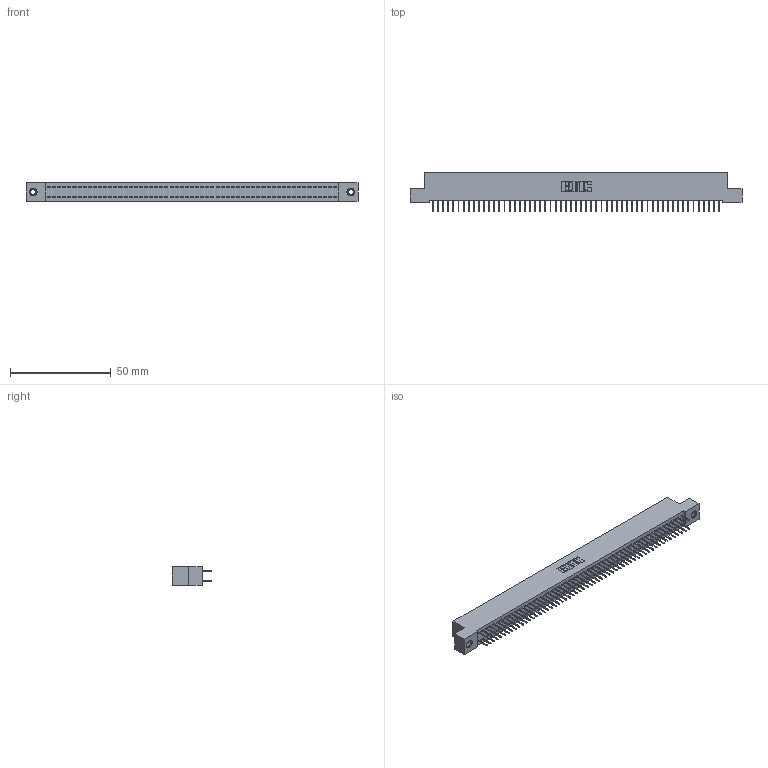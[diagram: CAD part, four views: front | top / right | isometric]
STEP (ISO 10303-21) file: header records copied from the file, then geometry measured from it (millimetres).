
FILE_DESCRIPTION (( 'STEP AP203' ), '1' );
FILE_NAME ('392-114-524-207.STEP', '2019-10-10T00:59:07', ( '' ), ( '' ), 'SwSTEP 2.0', 'SolidWorks 2016', '' );
FILE_SCHEMA (( 'CONFIG_CONTROL_DESIGN' ));
Length unit declared in the file: inch
Products named in the file (4): 345-250-001_345-250-005-103; 392-114-524-207; 342 Part_TI; 345-292-001_345-293-124
Assembly tree (117 placements, depth 2):
  392-114-524-207
    342 Part_TI
    345-292-001_345-293-124  x114
    345-250-001_345-250-005-103  x2
Bounding box: 165.1 x 19.69 x 9.4 mm (x, y, z)
Volume: 14720 mm3; surface area: 23907.1 mm2
Topology: 117 solids, 117 shells, 6554 faces, 18561 edges, 11910 vertices
Faces by surface type: plane 4886, cylinder 1652, cone 12, torus 4
Entity records: 35858 total; most frequent: CARTESIAN_POINT 5905, ORIENTED_EDGE 5834, DIRECTION 5051, EDGE_CURVE 2917, VECTOR 2773, LINE 2773, VERTEX_POINT 1936, AXIS2_PLACEMENT_3D 1139
